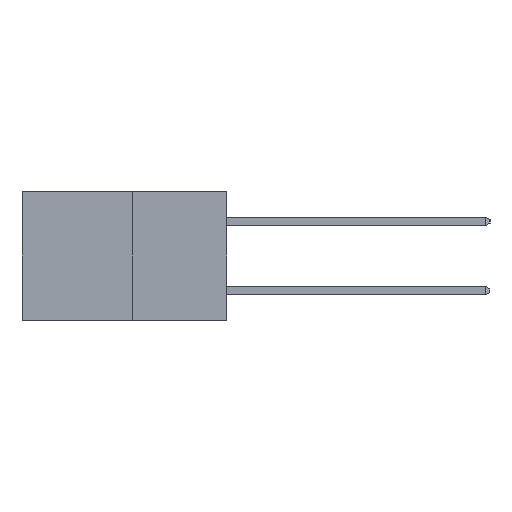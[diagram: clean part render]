
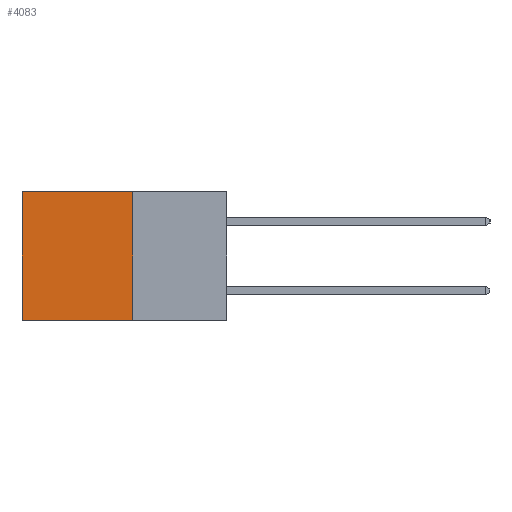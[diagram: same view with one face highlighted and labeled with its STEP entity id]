
A CAD part, left-side view. The second image highlights one B-rep face of the part: STEP entity #4083.
In plain terms, the highlighted planar face has unit normal (-1, 0, 0).
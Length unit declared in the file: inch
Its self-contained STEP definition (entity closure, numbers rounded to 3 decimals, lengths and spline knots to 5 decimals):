
#227 = EDGE_CURVE ( 'NONE', #9194, #538, #283, .T. ) ;
#283 = LINE ( 'NONE', #8909, #6094 ) ;
#538 = VERTEX_POINT ( 'NONE', #8379 ) ;
#957 = DIRECTION ( 'NONE',  ( 0., 0., -1. ) ) ;
#1030 = ORIENTED_EDGE ( 'NONE', *, *, #2372, .F. ) ;
#1510 = VECTOR ( 'NONE', #1557, 39.37008 ) ;
#1557 = DIRECTION ( 'NONE',  ( 0., 1., 0. ) ) ;
#1707 = VECTOR ( 'NONE', #1950, 39.37008 ) ;
#1946 = LINE ( 'NONE', #9166, #1707 ) ;
#1950 = DIRECTION ( 'NONE',  ( 0., 0., -1. ) ) ;
#2102 = EDGE_LOOP ( 'NONE', ( #4170, #9046, #1030, #3858 ) ) ;
#2372 = EDGE_CURVE ( 'NONE', #9194, #4954, #1946, .T. ) ;
#3046 = EDGE_CURVE ( 'NONE', #538, #3530, #9085, .T. ) ;
#3107 = FACE_OUTER_BOUND ( 'NONE', #2102, .T. ) ;
#3474 = AXIS2_PLACEMENT_3D ( 'NONE', #4307, #4205, #4180 ) ;
#3530 = VERTEX_POINT ( 'NONE', #6941 ) ;
#3756 = LINE ( 'NONE', #5331, #1510 ) ;
#3858 = ORIENTED_EDGE ( 'NONE', *, *, #227, .T. ) ;
#4083 = ADVANCED_FACE ( 'NONE', ( #3107 ), #4343, .F. ) ;
#4170 = ORIENTED_EDGE ( 'NONE', *, *, #3046, .T. ) ;
#4180 = DIRECTION ( 'NONE',  ( 0., 0., -1. ) ) ;
#4205 = DIRECTION ( 'NONE',  ( 1., 0., 0. ) ) ;
#4307 = CARTESIAN_POINT ( 'NONE',  ( 0.277, 0.27, -0.37 ) ) ;
#4343 = PLANE ( 'NONE',  #3474 ) ;
#4954 = VERTEX_POINT ( 'NONE', #7954 ) ;
#5189 = EDGE_CURVE ( 'NONE', #4954, #3530, #3756, .T. ) ;
#5261 = CARTESIAN_POINT ( 'NONE',  ( 0.277, 0.27, 0. ) ) ;
#5331 = CARTESIAN_POINT ( 'NONE',  ( 0.277, 0.27, -0.37 ) ) ;
#5356 = VECTOR ( 'NONE', #957, 39.37008 ) ;
#6094 = VECTOR ( 'NONE', #9246, 39.37008 ) ;
#6941 = CARTESIAN_POINT ( 'NONE',  ( 0.277, 0.59, -0.37 ) ) ;
#7954 = CARTESIAN_POINT ( 'NONE',  ( 0.277, 0.27, -0.37 ) ) ;
#8379 = CARTESIAN_POINT ( 'NONE',  ( 0.277, 0.59, 0. ) ) ;
#8909 = CARTESIAN_POINT ( 'NONE',  ( 0.277, 0.27, 0. ) ) ;
#9046 = ORIENTED_EDGE ( 'NONE', *, *, #5189, .F. ) ;
#9085 = LINE ( 'NONE', #9117, #5356 ) ;
#9117 = CARTESIAN_POINT ( 'NONE',  ( 0.277, 0.59, -0.37 ) ) ;
#9166 = CARTESIAN_POINT ( 'NONE',  ( 0.277, 0.27, -0.37 ) ) ;
#9194 = VERTEX_POINT ( 'NONE', #5261 ) ;
#9246 = DIRECTION ( 'NONE',  ( 0., 1., 0. ) ) ;
